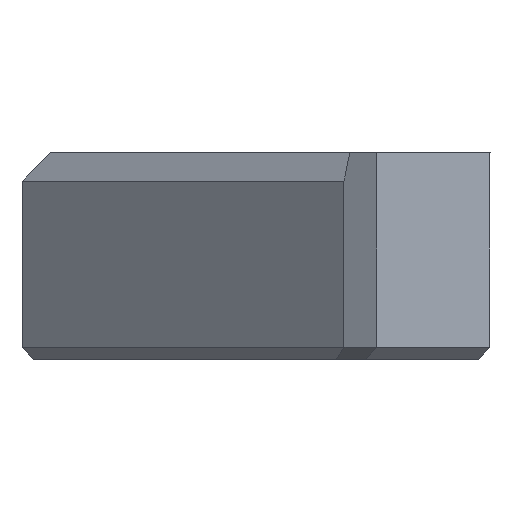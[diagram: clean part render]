
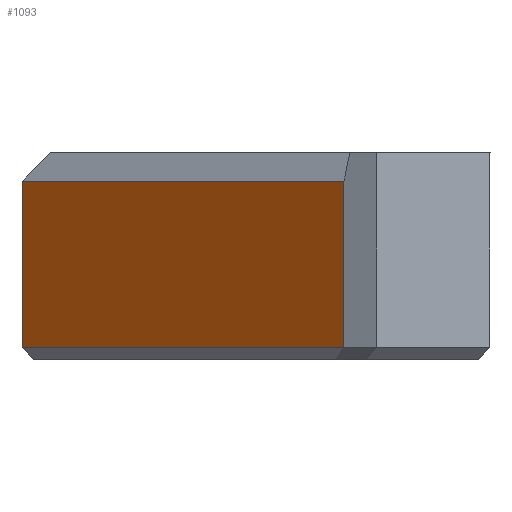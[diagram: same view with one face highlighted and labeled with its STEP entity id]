
A CAD part, left-side view. The second image highlights one B-rep face of the part: STEP entity #1093.
In plain terms, the highlighted planar face has unit normal (-0.73, 0.683, 0).
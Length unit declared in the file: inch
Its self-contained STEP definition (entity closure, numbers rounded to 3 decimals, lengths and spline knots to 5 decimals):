
#11 = DIRECTION ( 'NONE',  ( 0., 0., 1. ) ) ;
#28 = CARTESIAN_POINT ( 'NONE',  ( -4.91753, 1.3998, 3.40822 ) ) ;
#46 = EDGE_CURVE ( 'NONE', #146, #461, #471, .T. ) ;
#53 = CARTESIAN_POINT ( 'NONE',  ( -4.91753, 1.3998, 1.21096 ) ) ;
#58 = VERTEX_POINT ( 'NONE', #415 ) ;
#79 = VERTEX_POINT ( 'NONE', #28 ) ;
#92 = VECTOR ( 'NONE', #522, 39.37008 ) ;
#105 = CARTESIAN_POINT ( 'NONE',  ( -4.52124, 1.823, 1.21096 ) ) ;
#112 = LINE ( 'NONE', #105, #1127 ) ;
#146 = VERTEX_POINT ( 'NONE', #513 ) ;
#151 = FACE_OUTER_BOUND ( 'NONE', #243, .T. ) ;
#243 = EDGE_LOOP ( 'NONE', ( #867, #805, #955, #282 ) ) ;
#248 = VECTOR ( 'NONE', #537, 39.37008 ) ;
#282 = ORIENTED_EDGE ( 'NONE', *, *, #46, .T. ) ;
#324 = EDGE_CURVE ( 'NONE', #146, #79, #862, .T. ) ;
#340 = CARTESIAN_POINT ( 'NONE',  ( -4.92154, 1.39551, 1.21096 ) ) ;
#347 = EDGE_CURVE ( 'NONE', #58, #79, #950, .T. ) ;
#415 = CARTESIAN_POINT ( 'NONE',  ( -4.52124, 1.823, 3.40822 ) ) ;
#437 = DIRECTION ( 'NONE',  ( 0., 0., -1. ) ) ;
#461 = VERTEX_POINT ( 'NONE', #791 ) ;
#471 = LINE ( 'NONE', #1210, #92 ) ;
#513 = CARTESIAN_POINT ( 'NONE',  ( -4.91753, 1.3998, 3.62697 ) ) ;
#522 = DIRECTION ( 'NONE',  ( 0.684, 0.73, 0. ) ) ;
#537 = DIRECTION ( 'NONE',  ( -0.684, -0.73, 0. ) ) ;
#681 = VECTOR ( 'NONE', #437, 39.37008 ) ;
#751 = DIRECTION ( 'NONE',  ( -0.73, 0.684, 0. ) ) ;
#791 = CARTESIAN_POINT ( 'NONE',  ( -4.52124, 1.823, 3.62697 ) ) ;
#805 = ORIENTED_EDGE ( 'NONE', *, *, #347, .T. ) ;
#862 = LINE ( 'NONE', #53, #681 ) ;
#867 = ORIENTED_EDGE ( 'NONE', *, *, #1269, .F. ) ;
#938 = PLANE ( 'NONE',  #1217 ) ;
#950 = LINE ( 'NONE', #1125, #248 ) ;
#955 = ORIENTED_EDGE ( 'NONE', *, *, #324, .F. ) ;
#1038 = DIRECTION ( 'NONE',  ( 0.684, 0.73, 0. ) ) ;
#1093 = ADVANCED_FACE ( 'NONE', ( #151 ), #938, .T. ) ;
#1125 = CARTESIAN_POINT ( 'NONE',  ( -4.91753, 1.3998, 3.40822 ) ) ;
#1127 = VECTOR ( 'NONE', #11, 39.37008 ) ;
#1210 = CARTESIAN_POINT ( 'NONE',  ( -4.52124, 1.823, 3.62697 ) ) ;
#1217 = AXIS2_PLACEMENT_3D ( 'NONE', #340, #751, #1038 ) ;
#1269 = EDGE_CURVE ( 'NONE', #58, #461, #112, .T. ) ;
